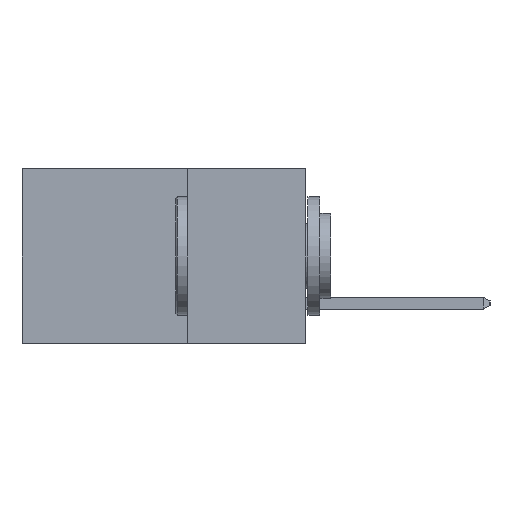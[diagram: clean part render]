
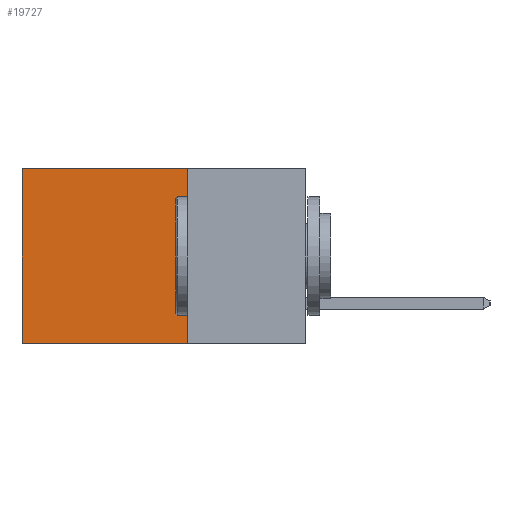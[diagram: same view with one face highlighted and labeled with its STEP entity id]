
A CAD part, left-side view. The second image highlights one B-rep face of the part: STEP entity #19727.
In plain terms, the highlighted planar face has unit normal (-1, 0, 0).
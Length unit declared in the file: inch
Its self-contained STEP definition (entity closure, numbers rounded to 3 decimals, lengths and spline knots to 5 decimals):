
#565 = AXIS2_PLACEMENT_3D ( 'NONE', #5609, #7383, #19060 ) ;
#1510 = EDGE_CURVE ( 'NONE', #7543, #18982, #16980, .T. ) ;
#1970 = VERTEX_POINT ( 'NONE', #20407 ) ;
#1992 = ORIENTED_EDGE ( 'NONE', *, *, #13632, .T. ) ;
#2536 = DIRECTION ( 'NONE',  ( 0., 1., 0. ) ) ;
#3052 = CARTESIAN_POINT ( 'NONE',  ( 0.2615, 0.25, -0.37 ) ) ;
#3221 = ORIENTED_EDGE ( 'NONE', *, *, #3606, .T. ) ;
#3606 = EDGE_CURVE ( 'NONE', #13128, #18982, #17932, .T. ) ;
#3970 = DIRECTION ( 'NONE',  ( 0., 0., -1. ) ) ;
#4063 = CARTESIAN_POINT ( 'NONE',  ( 0.2615, 0.6, -0.37 ) ) ;
#5609 = CARTESIAN_POINT ( 'NONE',  ( 0.2615, 0.25, -0.37 ) ) ;
#6308 = EDGE_CURVE ( 'NONE', #1970, #7543, #20599, .T. ) ;
#6532 = VECTOR ( 'NONE', #14135, 39.37008 ) ;
#7117 = CARTESIAN_POINT ( 'NONE',  ( 0.2615, 0.6, -0.37 ) ) ;
#7157 = DIRECTION ( 'NONE',  ( 0., 0., -1. ) ) ;
#7179 = CARTESIAN_POINT ( 'NONE',  ( 0.2615, 0.25, -0.37 ) ) ;
#7383 = DIRECTION ( 'NONE',  ( 1., 0., 0. ) ) ;
#7543 = VERTEX_POINT ( 'NONE', #20993 ) ;
#8985 = PLANE ( 'NONE',  #565 ) ;
#9040 = VECTOR ( 'NONE', #3970, 39.37008 ) ;
#10322 = FACE_OUTER_BOUND ( 'NONE', #18051, .T. ) ;
#11041 = LINE ( 'NONE', #17425, #6532 ) ;
#11328 = CARTESIAN_POINT ( 'NONE',  ( 0.2615, 0.6, 0. ) ) ;
#13128 = VERTEX_POINT ( 'NONE', #11328 ) ;
#13632 = EDGE_CURVE ( 'NONE', #1970, #13128, #11041, .T. ) ;
#14135 = DIRECTION ( 'NONE',  ( 0., 1., 0. ) ) ;
#15932 = VECTOR ( 'NONE', #2536, 39.37008 ) ;
#15962 = ORIENTED_EDGE ( 'NONE', *, *, #1510, .F. ) ;
#16980 = LINE ( 'NONE', #3052, #15932 ) ;
#17425 = CARTESIAN_POINT ( 'NONE',  ( 0.2615, 0.25, 0. ) ) ;
#17932 = LINE ( 'NONE', #4063, #9040 ) ;
#18051 = EDGE_LOOP ( 'NONE', ( #3221, #15962, #18427, #1992 ) ) ;
#18427 = ORIENTED_EDGE ( 'NONE', *, *, #6308, .F. ) ;
#18982 = VERTEX_POINT ( 'NONE', #7117 ) ;
#19060 = DIRECTION ( 'NONE',  ( 0., 0., -1. ) ) ;
#19603 = VECTOR ( 'NONE', #7157, 39.37008 ) ;
#19727 = ADVANCED_FACE ( 'NONE', ( #10322 ), #8985, .F. ) ;
#20407 = CARTESIAN_POINT ( 'NONE',  ( 0.2615, 0.25, 0. ) ) ;
#20599 = LINE ( 'NONE', #7179, #19603 ) ;
#20993 = CARTESIAN_POINT ( 'NONE',  ( 0.2615, 0.25, -0.37 ) ) ;
